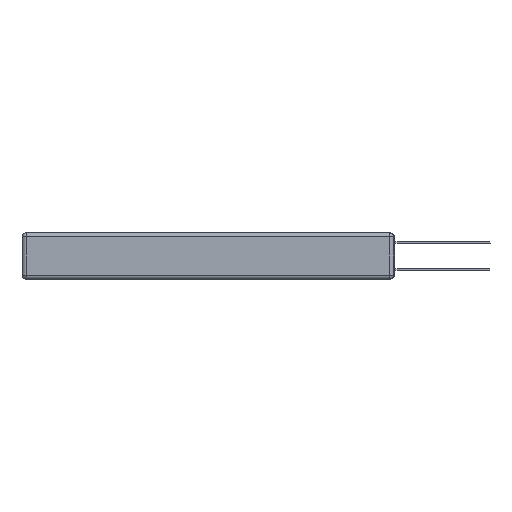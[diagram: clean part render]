
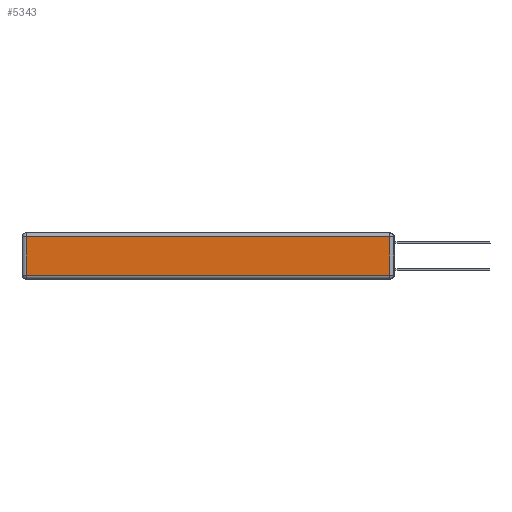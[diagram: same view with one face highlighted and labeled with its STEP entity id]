
A CAD part, left-side view. The second image highlights one B-rep face of the part: STEP entity #5343.
In plain terms, the highlighted planar face has unit normal (-1, 0, 0).
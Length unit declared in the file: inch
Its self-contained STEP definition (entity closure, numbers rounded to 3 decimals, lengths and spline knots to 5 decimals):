
#233 = CARTESIAN_POINT ( 'NONE',  ( 0., 2.75, -0.03 ) ) ;
#1548 = EDGE_CURVE ( 'NONE', #9814, #2237, #16436, .T. ) ;
#2237 = VERTEX_POINT ( 'NONE', #13408 ) ;
#2292 = DIRECTION ( 'NONE',  ( 0., -1., 0. ) ) ;
#2884 = CARTESIAN_POINT ( 'NONE',  ( 0., 0., -0.343 ) ) ;
#3656 = AXIS2_PLACEMENT_3D ( 'NONE', #2884, #7220, #4834 ) ;
#4834 = DIRECTION ( 'NONE',  ( 0., 0., 1. ) ) ;
#5343 = ADVANCED_FACE ( 'NONE', ( #10729 ), #7031, .T. ) ;
#6061 = DIRECTION ( 'NONE',  ( 0., 1., 0. ) ) ;
#6556 = VECTOR ( 'NONE', #2292, 39.37008 ) ;
#7031 = PLANE ( 'NONE',  #3656 ) ;
#7109 = EDGE_CURVE ( 'NONE', #2237, #12628, #7453, .T. ) ;
#7220 = DIRECTION ( 'NONE',  ( -1., 0., 0. ) ) ;
#7453 = LINE ( 'NONE', #233, #17973 ) ;
#7800 = ORIENTED_EDGE ( 'NONE', *, *, #21532, .T. ) ;
#8693 = VERTEX_POINT ( 'NONE', #19410 ) ;
#9814 = VERTEX_POINT ( 'NONE', #23502 ) ;
#10085 = VECTOR ( 'NONE', #14292, 39.37008 ) ;
#10729 = FACE_OUTER_BOUND ( 'NONE', #15506, .T. ) ;
#11773 = CARTESIAN_POINT ( 'NONE',  ( 0., 2.72, -0.03 ) ) ;
#12017 = LINE ( 'NONE', #24684, #6556 ) ;
#12628 = VERTEX_POINT ( 'NONE', #11773 ) ;
#13408 = CARTESIAN_POINT ( 'NONE',  ( 0., 0.03, -0.03 ) ) ;
#14292 = DIRECTION ( 'NONE',  ( 0., 0., 1. ) ) ;
#14928 = ORIENTED_EDGE ( 'NONE', *, *, #1548, .T. ) ;
#15506 = EDGE_LOOP ( 'NONE', ( #21921, #14928, #23751, #7800 ) ) ;
#16436 = LINE ( 'NONE', #24495, #10085 ) ;
#16706 = CARTESIAN_POINT ( 'NONE',  ( 0., 2.72, -0.343 ) ) ;
#17973 = VECTOR ( 'NONE', #6061, 39.37008 ) ;
#18201 = EDGE_CURVE ( 'NONE', #8693, #9814, #12017, .T. ) ;
#18755 = DIRECTION ( 'NONE',  ( 0., 0., -1. ) ) ;
#19146 = LINE ( 'NONE', #16706, #23606 ) ;
#19410 = CARTESIAN_POINT ( 'NONE',  ( 0., 2.72, -0.313 ) ) ;
#21532 = EDGE_CURVE ( 'NONE', #12628, #8693, #19146, .T. ) ;
#21921 = ORIENTED_EDGE ( 'NONE', *, *, #18201, .T. ) ;
#23502 = CARTESIAN_POINT ( 'NONE',  ( 0., 0.03, -0.313 ) ) ;
#23606 = VECTOR ( 'NONE', #18755, 39.37008 ) ;
#23751 = ORIENTED_EDGE ( 'NONE', *, *, #7109, .T. ) ;
#24495 = CARTESIAN_POINT ( 'NONE',  ( 0., 0.03, -0.343 ) ) ;
#24684 = CARTESIAN_POINT ( 'NONE',  ( 0., 0., -0.313 ) ) ;
